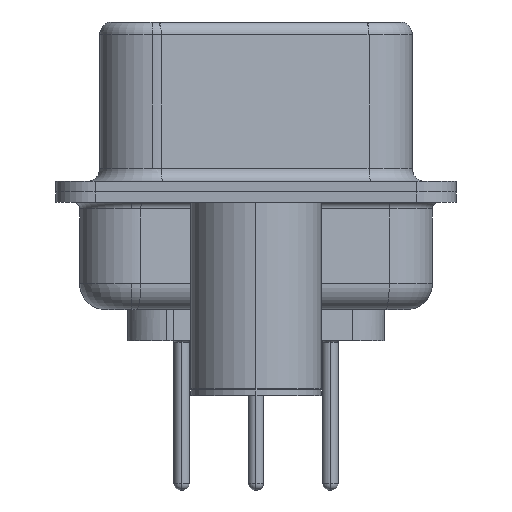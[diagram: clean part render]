
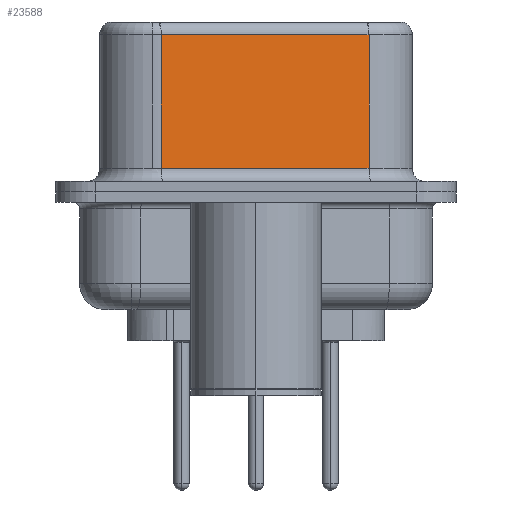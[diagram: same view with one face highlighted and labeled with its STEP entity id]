
A CAD part, left-side view. The second image highlights one B-rep face of the part: STEP entity #23588.
In plain terms, the highlighted planar face has unit normal (-0.985, -0.174, 0).
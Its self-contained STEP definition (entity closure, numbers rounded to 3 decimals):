
#226 = ORIENTED_EDGE ( 'NONE', *, *, #18382, .T. ) ;
#3420 = VERTEX_POINT ( 'NONE', #8033 ) ;
#4037 = ORIENTED_EDGE ( 'NONE', *, *, #4987, .F. ) ;
#4987 = EDGE_CURVE ( 'NONE', #28370, #7575, #27422, .T. ) ;
#5191 = CARTESIAN_POINT ( 'NONE',  ( 3.73, 3.628, 6.52 ) ) ;
#5307 = DIRECTION ( 'NONE',  ( 0.174, -0.985, 0. ) ) ;
#5570 = CARTESIAN_POINT ( 'NONE',  ( 5.132, -4.322, 6.02 ) ) ;
#5608 = DIRECTION ( 'NONE',  ( -0.174, 0.985, 0. ) ) ;
#7575 = VERTEX_POINT ( 'NONE', #27502 ) ;
#7625 = CARTESIAN_POINT ( 'NONE',  ( 3.73, 3.628, 6.02 ) ) ;
#8033 = CARTESIAN_POINT ( 'NONE',  ( 3.73, 3.628, 0.9 ) ) ;
#9422 = VECTOR ( 'NONE', #25834, 1000. ) ;
#9753 = LINE ( 'NONE', #5191, #28008 ) ;
#9941 = VECTOR ( 'NONE', #5307, 1000. ) ;
#10707 = EDGE_CURVE ( 'NONE', #16716, #3420, #9753, .T. ) ;
#13021 = DIRECTION ( 'NONE',  ( 0.985, 0.174, 0. ) ) ;
#15144 = FACE_OUTER_BOUND ( 'NONE', #23630, .T. ) ;
#15289 = CARTESIAN_POINT ( 'NONE',  ( 5.132, -4.322, 6.52 ) ) ;
#16716 = VERTEX_POINT ( 'NONE', #7625 ) ;
#17818 = EDGE_CURVE ( 'NONE', #28370, #16716, #19166, .T. ) ;
#18382 = EDGE_CURVE ( 'NONE', #3420, #7575, #19719, .T. ) ;
#18972 = AXIS2_PLACEMENT_3D ( 'NONE', #23966, #13021, #5608 ) ;
#19166 = LINE ( 'NONE', #28401, #9422 ) ;
#19719 = LINE ( 'NONE', #21705, #9941 ) ;
#20449 = ORIENTED_EDGE ( 'NONE', *, *, #17818, .T. ) ;
#21705 = CARTESIAN_POINT ( 'NONE',  ( 5.132, -4.322, 0.9 ) ) ;
#23588 = ADVANCED_FACE ( 'NONE', ( #15144 ), #26675, .F. ) ;
#23630 = EDGE_LOOP ( 'NONE', ( #4037, #20449, #29354, #226 ) ) ;
#23696 = DIRECTION ( 'NONE',  ( 0., 0., -1. ) ) ;
#23966 = CARTESIAN_POINT ( 'NONE',  ( 5.132, -4.322, 6.52 ) ) ;
#24836 = DIRECTION ( 'NONE',  ( 0., 0., -1. ) ) ;
#25210 = VECTOR ( 'NONE', #24836, 1000. ) ;
#25834 = DIRECTION ( 'NONE',  ( -0.174, 0.985, 0. ) ) ;
#26675 = PLANE ( 'NONE',  #18972 ) ;
#27422 = LINE ( 'NONE', #15289, #25210 ) ;
#27502 = CARTESIAN_POINT ( 'NONE',  ( 5.132, -4.322, 0.9 ) ) ;
#28008 = VECTOR ( 'NONE', #23696, 1000. ) ;
#28370 = VERTEX_POINT ( 'NONE', #5570 ) ;
#28401 = CARTESIAN_POINT ( 'NONE',  ( 5.132, -4.322, 6.02 ) ) ;
#29354 = ORIENTED_EDGE ( 'NONE', *, *, #10707, .T. ) ;
